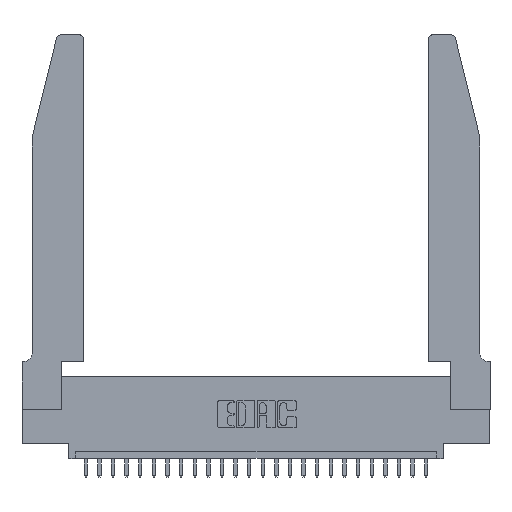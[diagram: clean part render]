
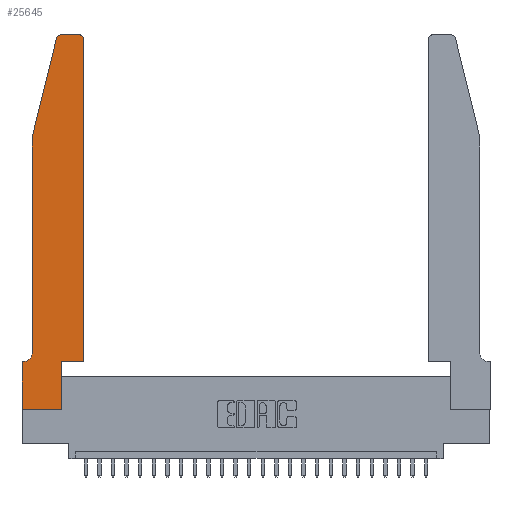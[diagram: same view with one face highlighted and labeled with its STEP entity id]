
A CAD part, top view. The second image highlights one B-rep face of the part: STEP entity #25645.
In plain terms, the highlighted planar face has unit normal (0, 0, 1).
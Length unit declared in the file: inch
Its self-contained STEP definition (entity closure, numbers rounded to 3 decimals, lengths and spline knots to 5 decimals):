
#121 = CARTESIAN_POINT ( 'NONE',  ( 0.0055, 0.35, 0.37 ) ) ;
#279 = CARTESIAN_POINT ( 'NONE',  ( 0.0755, 2., 0.37 ) ) ;
#328 = ORIENTED_EDGE ( 'NONE', *, *, #23827, .T. ) ;
#638 = CARTESIAN_POINT ( 'NONE',  ( 0.2865, 0.35, 0.37 ) ) ;
#829 = DIRECTION ( 'NONE',  ( 0., 0., 1. ) ) ;
#835 = CIRCLE ( 'NONE', #18074, 0.07 ) ;
#939 = ORIENTED_EDGE ( 'NONE', *, *, #2711, .T. ) ;
#1410 = VERTEX_POINT ( 'NONE', #14535 ) ;
#2213 = CARTESIAN_POINT ( 'NONE',  ( 0., 0.35, 0.37 ) ) ;
#2308 = CIRCLE ( 'NONE', #20971, 0.03 ) ;
#2711 = EDGE_CURVE ( 'NONE', #15138, #19319, #19928, .T. ) ;
#2799 = AXIS2_PLACEMENT_3D ( 'NONE', #11364, #829, #25708 ) ;
#2926 = CARTESIAN_POINT ( 'NONE',  ( 0.4505, 2.72, 0.37 ) ) ;
#3166 = LINE ( 'NONE', #24421, #13827 ) ;
#3333 = VECTOR ( 'NONE', #4160, 39.37008 ) ;
#3526 = VECTOR ( 'NONE', #6382, 39.37008 ) ;
#3648 = ORIENTED_EDGE ( 'NONE', *, *, #4866, .T. ) ;
#3800 = CIRCLE ( 'NONE', #2799, 0.03 ) ;
#4160 = DIRECTION ( 'NONE',  ( 0., -1., 0. ) ) ;
#4363 = ORIENTED_EDGE ( 'NONE', *, *, #15733, .T. ) ;
#4763 = CARTESIAN_POINT ( 'NONE',  ( 0.25487, 2.72718, 0.37 ) ) ;
#4866 = EDGE_CURVE ( 'NONE', #5568, #16201, #24673, .T. ) ;
#4981 = ORIENTED_EDGE ( 'NONE', *, *, #12369, .T. ) ;
#5296 = CARTESIAN_POINT ( 'NONE',  ( 0.0755, 0.35, 0.37 ) ) ;
#5393 = DIRECTION ( 'NONE',  ( 0., 1., 0. ) ) ;
#5480 = DIRECTION ( 'NONE',  ( -1., 0., 0. ) ) ;
#5502 = LINE ( 'NONE', #638, #12943 ) ;
#5568 = VERTEX_POINT ( 'NONE', #12228 ) ;
#5633 = VERTEX_POINT ( 'NONE', #11951 ) ;
#6114 = ORIENTED_EDGE ( 'NONE', *, *, #20479, .T. ) ;
#6382 = DIRECTION ( 'NONE',  ( 1., 0., 0. ) ) ;
#6559 = DIRECTION ( 'NONE',  ( -0.239, -0.971, 0. ) ) ;
#6705 = AXIS2_PLACEMENT_3D ( 'NONE', #7005, #10901, #8824 ) ;
#6954 = EDGE_CURVE ( 'NONE', #16201, #22243, #3800, .T. ) ;
#7005 = CARTESIAN_POINT ( 'NONE',  ( 0., 0.35, 0.37 ) ) ;
#7606 = VECTOR ( 'NONE', #21391, 39.37008 ) ;
#8824 = DIRECTION ( 'NONE',  ( 1., 0., 0. ) ) ;
#8864 = LINE ( 'NONE', #279, #3333 ) ;
#9088 = PLANE ( 'NONE',  #6705 ) ;
#9219 = LINE ( 'NONE', #25403, #7606 ) ;
#9357 = LINE ( 'NONE', #12348, #20617 ) ;
#9743 = CARTESIAN_POINT ( 'NONE',  ( 0.0755, 2., 0.37 ) ) ;
#10504 = DIRECTION ( 'NONE',  ( 0., 0., 1. ) ) ;
#10594 = CARTESIAN_POINT ( 'NONE',  ( 0.4205, 2.72, 0.37 ) ) ;
#10667 = DIRECTION ( 'NONE',  ( 0., 1., 0. ) ) ;
#10835 = CARTESIAN_POINT ( 'NONE',  ( 0.0055, 0.42, 0.37 ) ) ;
#10901 = DIRECTION ( 'NONE',  ( 0., 0., 1. ) ) ;
#11202 = CARTESIAN_POINT ( 'NONE',  ( 0.4505, 0.35, 0.37 ) ) ;
#11364 = CARTESIAN_POINT ( 'NONE',  ( 0.284, 2.72, 0.37 ) ) ;
#11549 = DIRECTION ( 'NONE',  ( -1., 0., 0. ) ) ;
#11951 = CARTESIAN_POINT ( 'NONE',  ( 0.2865, 0.35, 0.37 ) ) ;
#12228 = CARTESIAN_POINT ( 'NONE',  ( 0.4205, 2.75, 0.37 ) ) ;
#12348 = CARTESIAN_POINT ( 'NONE',  ( 0.0755, 2., 0.37 ) ) ;
#12369 = EDGE_CURVE ( 'NONE', #5633, #20112, #25414, .T. ) ;
#12710 = ORIENTED_EDGE ( 'NONE', *, *, #19897, .T. ) ;
#12943 = VECTOR ( 'NONE', #10667, 39.37008 ) ;
#13129 = CARTESIAN_POINT ( 'NONE',  ( 0., 0., 0.37 ) ) ;
#13225 = EDGE_LOOP ( 'NONE', ( #3648, #15761, #23322, #16742, #328, #939, #25885, #21748, #6114, #4981, #4363, #12710 ) ) ;
#13529 = CARTESIAN_POINT ( 'NONE',  ( 0.2605, 2.75, 0.37 ) ) ;
#13818 = EDGE_CURVE ( 'NONE', #19319, #19407, #9219, .T. ) ;
#13827 = VECTOR ( 'NONE', #22191, 39.37008 ) ;
#14484 = CARTESIAN_POINT ( 'NONE',  ( 0.4505, 0.35, 0.37 ) ) ;
#14535 = CARTESIAN_POINT ( 'NONE',  ( 0.0755, 0.42, 0.37 ) ) ;
#15138 = VERTEX_POINT ( 'NONE', #121 ) ;
#15432 = VERTEX_POINT ( 'NONE', #9743 ) ;
#15733 = EDGE_CURVE ( 'NONE', #20112, #25716, #15894, .T. ) ;
#15761 = ORIENTED_EDGE ( 'NONE', *, *, #6954, .T. ) ;
#15894 = LINE ( 'NONE', #19601, #22956 ) ;
#16201 = VERTEX_POINT ( 'NONE', #16203 ) ;
#16203 = CARTESIAN_POINT ( 'NONE',  ( 0.284, 2.75, 0.37 ) ) ;
#16742 = ORIENTED_EDGE ( 'NONE', *, *, #25018, .T. ) ;
#17097 = DIRECTION ( 'NONE',  ( 0., 0., -1. ) ) ;
#18074 = AXIS2_PLACEMENT_3D ( 'NONE', #10835, #17097, #24919 ) ;
#19246 = VECTOR ( 'NONE', #5480, 39.37008 ) ;
#19319 = VERTEX_POINT ( 'NONE', #2213 ) ;
#19407 = VERTEX_POINT ( 'NONE', #13129 ) ;
#19601 = CARTESIAN_POINT ( 'NONE',  ( 0.4505, 0.35, 0.37 ) ) ;
#19602 = VECTOR ( 'NONE', #11549, 39.37008 ) ;
#19897 = EDGE_CURVE ( 'NONE', #25716, #5568, #2308, .T. ) ;
#19928 = LINE ( 'NONE', #5296, #19602 ) ;
#20112 = VERTEX_POINT ( 'NONE', #11202 ) ;
#20479 = EDGE_CURVE ( 'NONE', #26643, #5633, #5502, .T. ) ;
#20617 = VECTOR ( 'NONE', #6559, 39.37008 ) ;
#20971 = AXIS2_PLACEMENT_3D ( 'NONE', #10594, #10504, #23064 ) ;
#21082 = EDGE_CURVE ( 'NONE', #22243, #15432, #9357, .T. ) ;
#21391 = DIRECTION ( 'NONE',  ( 0., -1., 0. ) ) ;
#21457 = EDGE_CURVE ( 'NONE', #19407, #26643, #3166, .T. ) ;
#21748 = ORIENTED_EDGE ( 'NONE', *, *, #21457, .T. ) ;
#22191 = DIRECTION ( 'NONE',  ( 1., 0., 0. ) ) ;
#22243 = VERTEX_POINT ( 'NONE', #4763 ) ;
#22956 = VECTOR ( 'NONE', #5393, 39.37008 ) ;
#23064 = DIRECTION ( 'NONE',  ( 1., 0., 0. ) ) ;
#23322 = ORIENTED_EDGE ( 'NONE', *, *, #21082, .T. ) ;
#23827 = EDGE_CURVE ( 'NONE', #1410, #15138, #835, .T. ) ;
#24421 = CARTESIAN_POINT ( 'NONE',  ( 0., 0., 0.37 ) ) ;
#24673 = LINE ( 'NONE', #13529, #19246 ) ;
#24919 = DIRECTION ( 'NONE',  ( -1., 0., 0. ) ) ;
#25018 = EDGE_CURVE ( 'NONE', #15432, #1410, #8864, .T. ) ;
#25403 = CARTESIAN_POINT ( 'NONE',  ( 0., 0., 0.37 ) ) ;
#25414 = LINE ( 'NONE', #14484, #3526 ) ;
#25508 = FACE_OUTER_BOUND ( 'NONE', #13225, .T. ) ;
#25645 = ADVANCED_FACE ( 'NONE', ( #25508 ), #9088, .T. ) ;
#25708 = DIRECTION ( 'NONE',  ( 1., 0., 0. ) ) ;
#25716 = VERTEX_POINT ( 'NONE', #2926 ) ;
#25885 = ORIENTED_EDGE ( 'NONE', *, *, #13818, .T. ) ;
#26532 = CARTESIAN_POINT ( 'NONE',  ( 0.2865, 0., 0.37 ) ) ;
#26643 = VERTEX_POINT ( 'NONE', #26532 ) ;
